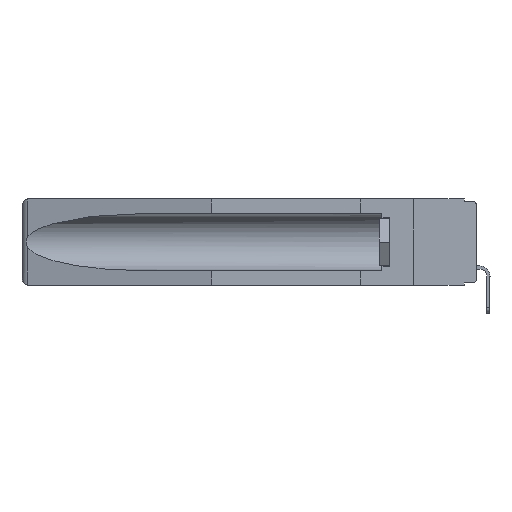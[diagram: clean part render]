
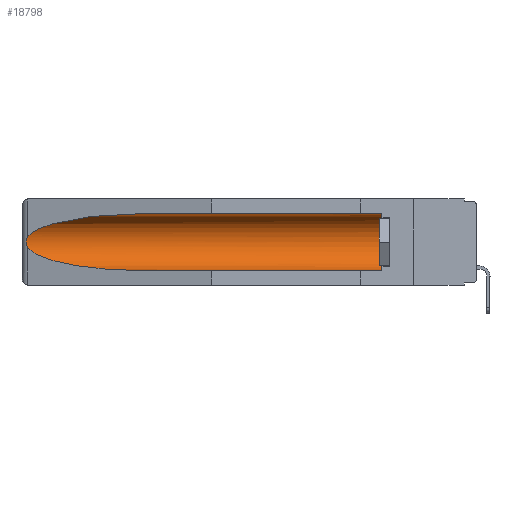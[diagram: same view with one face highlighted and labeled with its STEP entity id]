
A CAD part, left-side view. The second image highlights one B-rep face of the part: STEP entity #18798.
In plain terms, the highlighted cylindrical face has radius 2.857 mm (diameter 5.715 mm), a partial arc.
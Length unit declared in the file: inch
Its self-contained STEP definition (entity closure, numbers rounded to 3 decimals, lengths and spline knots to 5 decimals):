
#186 = DIRECTION ( 'NONE',  ( 0., 0., 1. ) ) ;
#1063 = CARTESIAN_POINT ( 'NONE',  ( 0.155, 1.07973, -0.059 ) ) ;
#1256 = CIRCLE ( 'NONE', #12232, 0.1125 ) ;
#1357 = CARTESIAN_POINT ( 'NONE',  ( 0.25451, 1.48313, -0.09465 ) ) ;
#1834 = CARTESIAN_POINT ( 'NONE',  ( 0.26537, 1.52718, -0.14972 ) ) ;
#2517 = ORIENTED_EDGE ( 'NONE', *, *, #9627, .T. ) ;
#2712 = CARTESIAN_POINT ( 'NONE',  ( 0.155, -0.30754, -0.1715 ) ) ;
#2850 = FACE_OUTER_BOUND ( 'NONE', #20977, .T. ) ;
#3144 = DIRECTION ( 'NONE',  ( 0., 1., 0. ) ) ;
#4005 = CARTESIAN_POINT ( 'NONE',  ( 0.25451, 1.48313, -0.24835 ) ) ;
#5486 = CARTESIAN_POINT ( 'NONE',  ( 0.26537, 1.52718, -0.14972 ) ) ;
#5492 = EDGE_CURVE ( 'NONE', #17495, #21509, #28316, .T. ) ;
#6149 = CARTESIAN_POINT ( 'NONE',  ( 0.26537, 1.52718, -0.19328 ) ) ;
#6417 = ORIENTED_EDGE ( 'NONE', *, *, #16914, .T. ) ;
#6951 = ORIENTED_EDGE ( 'NONE', *, *, #5492, .T. ) ;
#7089 = ORIENTED_EDGE ( 'NONE', *, *, #21248, .T. ) ;
#7482 = CARTESIAN_POINT ( 'NONE',  ( 0.155, -0.30754, -0.284 ) ) ;
#8350 = CARTESIAN_POINT ( 'NONE',  ( 0.26597, 1.5296, -0.19026 ) ) ;
#8484 = CARTESIAN_POINT ( 'NONE',  ( 0.2673, 1.53269, -0.17917 ) ) ;
#9627 = EDGE_CURVE ( 'NONE', #10082, #17495, #14267, .T. ) ;
#9891 = DIRECTION ( 'NONE',  ( 0., 1., 0. ) ) ;
#10082 = VERTEX_POINT ( 'NONE', #16899 ) ;
#10107 = VECTOR ( 'NONE', #9891, 39.37008 ) ;
#10770 = CARTESIAN_POINT ( 'NONE',  ( 0.2673, 1.5327, -0.16383 ) ) ;
#11516 =( BOUNDED_CURVE ( )  B_SPLINE_CURVE ( 3, ( #6149, #4005, #11783, #12737 ),
 .UNSPECIFIED., .F., .T. ) 
 B_SPLINE_CURVE_WITH_KNOTS ( ( 4, 4 ),
 ( 0.1948, 1.5708 ),
 .UNSPECIFIED. ) 
 CURVE ( )  GEOMETRIC_REPRESENTATION_ITEM ( )  RATIONAL_B_SPLINE_CURVE ( ( 1., 0.848, 0.848, 1. ) ) 
 REPRESENTATION_ITEM ( '' )  );
#11783 = CARTESIAN_POINT ( 'NONE',  ( 0.21114, 1.30732, -0.284 ) ) ;
#11793 = CARTESIAN_POINT ( 'NONE',  ( 0.155, 1.07973, -0.284 ) ) ;
#12039 = DIRECTION ( 'NONE',  ( 0., 1., 0. ) ) ;
#12179 = CARTESIAN_POINT ( 'NONE',  ( 0.155, 0.126, -0.284 ) ) ;
#12232 = AXIS2_PLACEMENT_3D ( 'NONE', #25991, #24240, #186 ) ;
#12320 = LINE ( 'NONE', #14172, #15206 ) ;
#12682 = ORIENTED_EDGE ( 'NONE', *, *, #13887, .T. ) ;
#12737 = CARTESIAN_POINT ( 'NONE',  ( 0.155, 1.07973, -0.284 ) ) ;
#13589 = CYLINDRICAL_SURFACE ( 'NONE', #16681, 0.1125 ) ;
#13640 = ORIENTED_EDGE ( 'NONE', *, *, #13943, .F. ) ;
#13887 = EDGE_CURVE ( 'NONE', #21509, #16389, #11516, .T. ) ;
#13943 = EDGE_CURVE ( 'NONE', #23449, #16389, #27095, .T. ) ;
#14172 = CARTESIAN_POINT ( 'NONE',  ( 0.155, -0.30754, -0.059 ) ) ;
#14179 = VERTEX_POINT ( 'NONE', #22451 ) ;
#14267 =( BOUNDED_CURVE ( )  B_SPLINE_CURVE ( 3, ( #1063, #23257, #1357, #5486 ),
 .UNSPECIFIED., .F., .T. ) 
 B_SPLINE_CURVE_WITH_KNOTS ( ( 4, 4 ),
 ( 4.71239, 6.08839 ),
 .UNSPECIFIED. ) 
 CURVE ( )  GEOMETRIC_REPRESENTATION_ITEM ( )  RATIONAL_B_SPLINE_CURVE ( ( 1., 0.848, 0.848, 1. ) ) 
 REPRESENTATION_ITEM ( '' )  );
#14331 = CARTESIAN_POINT ( 'NONE',  ( 0.26537, 1.52718, -0.19328 ) ) ;
#14499 = CARTESIAN_POINT ( 'NONE',  ( 0.26597, 1.52961, -0.15275 ) ) ;
#15206 = VECTOR ( 'NONE', #12039, 39.37008 ) ;
#16389 = VERTEX_POINT ( 'NONE', #11793 ) ;
#16681 = AXIS2_PLACEMENT_3D ( 'NONE', #2712, #3144, #22766 ) ;
#16899 = CARTESIAN_POINT ( 'NONE',  ( 0.155, 1.07973, -0.059 ) ) ;
#16914 = EDGE_CURVE ( 'NONE', #14179, #10082, #12320, .T. ) ;
#17495 = VERTEX_POINT ( 'NONE', #1834 ) ;
#18798 = ADVANCED_FACE ( 'NONE', ( #2850 ), #13589, .F. ) ;
#19243 = CARTESIAN_POINT ( 'NONE',  ( 0.26654, 1.53092, -0.15636 ) ) ;
#20977 = EDGE_LOOP ( 'NONE', ( #2517, #6951, #12682, #13640, #7089, #6417 ) ) ;
#21248 = EDGE_CURVE ( 'NONE', #23449, #14179, #1256, .T. ) ;
#21509 = VERTEX_POINT ( 'NONE', #14331 ) ;
#22451 = CARTESIAN_POINT ( 'NONE',  ( 0.155, 0.126, -0.059 ) ) ;
#22766 = DIRECTION ( 'NONE',  ( 0., 0., 1. ) ) ;
#23257 = CARTESIAN_POINT ( 'NONE',  ( 0.21114, 1.30732, -0.059 ) ) ;
#23449 = VERTEX_POINT ( 'NONE', #12179 ) ;
#23537 = CARTESIAN_POINT ( 'NONE',  ( 0.2675, 1.53308, -0.16763 ) ) ;
#24240 = DIRECTION ( 'NONE',  ( 0., -1., 0. ) ) ;
#25694 = CARTESIAN_POINT ( 'NONE',  ( 0.26537, 1.52718, -0.19328 ) ) ;
#25839 = CARTESIAN_POINT ( 'NONE',  ( 0.26655, 1.53094, -0.18657 ) ) ;
#25982 = CARTESIAN_POINT ( 'NONE',  ( 0.2675, 1.53308, -0.17534 ) ) ;
#25991 = CARTESIAN_POINT ( 'NONE',  ( 0.155, 0.126, -0.1715 ) ) ;
#27095 = LINE ( 'NONE', #7482, #10107 ) ;
#27961 = CARTESIAN_POINT ( 'NONE',  ( 0.26537, 1.52718, -0.14972 ) ) ;
#28316 = B_SPLINE_CURVE_WITH_KNOTS ( 'NONE', 3,
 ( #27961, #14499, #19243, #10770, #23537, #25982, #8484, #25839, #8350, #25694 ),
 .UNSPECIFIED., .F., .F.,
 ( 4, 2, 2, 2, 4 ),
 ( 0., 0.00029, 0.00058, 0.00087, 0.00117 ),
 .UNSPECIFIED. ) ;
